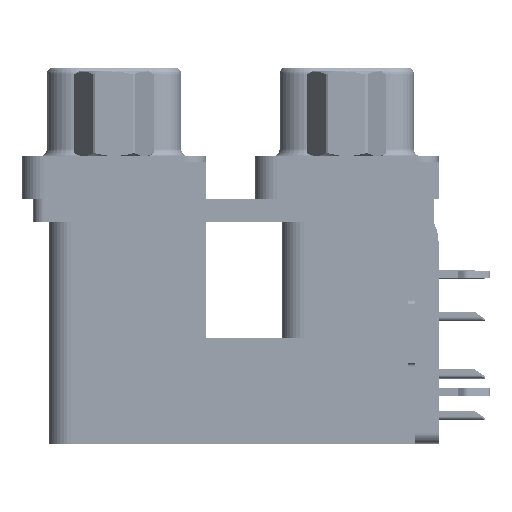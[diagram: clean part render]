
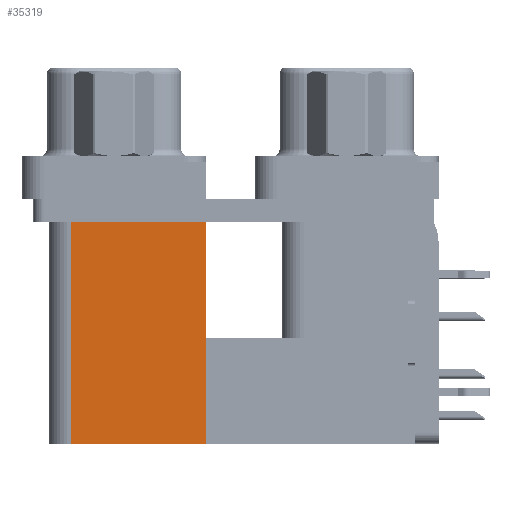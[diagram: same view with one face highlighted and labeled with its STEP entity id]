
A CAD part, left-side view. The second image highlights one B-rep face of the part: STEP entity #35319.
In plain terms, the highlighted planar face has unit normal (-1, 0, 0).
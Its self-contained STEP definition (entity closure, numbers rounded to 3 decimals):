
#464 = ORIENTED_EDGE ( 'NONE', *, *, #18133, .T. ) ;
#5097 = LINE ( 'NONE', #50798, #50917 ) ;
#8700 = VERTEX_POINT ( 'NONE', #51133 ) ;
#11700 = EDGE_LOOP ( 'NONE', ( #26318, #41898, #23190, #464 ) ) ;
#12730 = EDGE_CURVE ( 'NONE', #52092, #48128, #5097, .T. ) ;
#14508 = DIRECTION ( 'NONE',  ( 0., 0., 1. ) ) ;
#15549 = CARTESIAN_POINT ( 'NONE',  ( 3.79, 18.8, -2.5 ) ) ;
#15745 = DIRECTION ( 'NONE',  ( 0., 1., 0. ) ) ;
#17903 = VECTOR ( 'NONE', #15745, 1000. ) ;
#18133 = EDGE_CURVE ( 'NONE', #48087, #8700, #52232, .T. ) ;
#20428 = VECTOR ( 'NONE', #57253, 1000. ) ;
#20700 = LINE ( 'NONE', #42814, #20428 ) ;
#23190 = ORIENTED_EDGE ( 'NONE', *, *, #23364, .F. ) ;
#23364 = EDGE_CURVE ( 'NONE', #48087, #52092, #20700, .T. ) ;
#23703 = PLANE ( 'NONE',  #31879 ) ;
#26318 = ORIENTED_EDGE ( 'NONE', *, *, #42865, .T. ) ;
#28124 = CARTESIAN_POINT ( 'NONE',  ( 3.79, 9.6, -19.2 ) ) ;
#28417 = FACE_OUTER_BOUND ( 'NONE', #11700, .T. ) ;
#29896 = LINE ( 'NONE', #43465, #17903 ) ;
#31879 = AXIS2_PLACEMENT_3D ( 'NONE', #28124, #36671, #46385 ) ;
#34842 = CARTESIAN_POINT ( 'NONE',  ( 3.79, 9.6, -19.2 ) ) ;
#35319 = ADVANCED_FACE ( 'NONE', ( #28417 ), #23703, .F. ) ;
#36671 = DIRECTION ( 'NONE',  ( 1., 0., 0. ) ) ;
#41898 = ORIENTED_EDGE ( 'NONE', *, *, #12730, .F. ) ;
#42556 = CARTESIAN_POINT ( 'NONE',  ( 3.79, 18.8, -19.2 ) ) ;
#42814 = CARTESIAN_POINT ( 'NONE',  ( 3.79, 9.6, -19.2 ) ) ;
#42865 = EDGE_CURVE ( 'NONE', #8700, #48128, #29896, .T. ) ;
#43465 = CARTESIAN_POINT ( 'NONE',  ( 3.79, 9.6, -2.5 ) ) ;
#46385 = DIRECTION ( 'NONE',  ( 0., 0., -1. ) ) ;
#48087 = VERTEX_POINT ( 'NONE', #50953 ) ;
#48128 = VERTEX_POINT ( 'NONE', #15549 ) ;
#50224 = VECTOR ( 'NONE', #57541, 1000. ) ;
#50798 = CARTESIAN_POINT ( 'NONE',  ( 3.79, 18.8, -19.2 ) ) ;
#50917 = VECTOR ( 'NONE', #14508, 1000. ) ;
#50953 = CARTESIAN_POINT ( 'NONE',  ( 3.79, 9.6, -19.2 ) ) ;
#51133 = CARTESIAN_POINT ( 'NONE',  ( 3.79, 9.6, -2.5 ) ) ;
#52092 = VERTEX_POINT ( 'NONE', #42556 ) ;
#52232 = LINE ( 'NONE', #34842, #50224 ) ;
#57253 = DIRECTION ( 'NONE',  ( 0., 1., 0. ) ) ;
#57541 = DIRECTION ( 'NONE',  ( 0., 0., 1. ) ) ;
